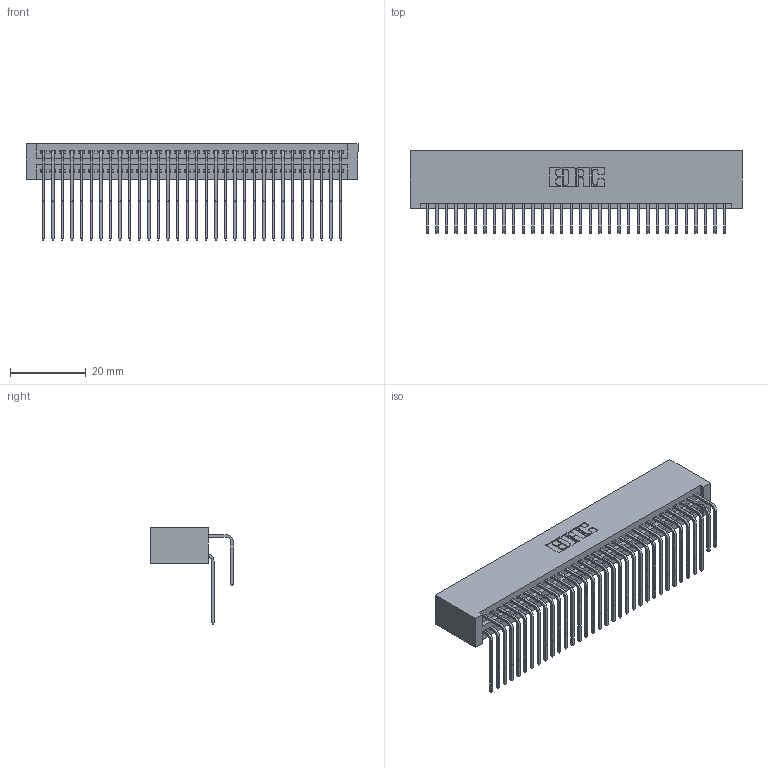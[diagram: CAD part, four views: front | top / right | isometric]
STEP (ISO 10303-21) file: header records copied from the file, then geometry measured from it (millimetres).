
FILE_DESCRIPTION (( 'STEP AP203' ), '1' );
FILE_NAME ('345-064-558-201.STEP', '2019-10-30T15:08:09', ( '' ), ( '' ), 'SwSTEP 2.0', 'SolidWorks 2016', '' );
FILE_SCHEMA (( 'CONFIG_CONTROL_DESIGN' ));
Length unit declared in the file: inch
Products named in the file (4): 345-292-001_558 Tail - 2; 345-292-001_558 559 Tail - 1; 345 Part_No Mounting Lugs; 345-064-558-201
Assembly tree (65 placements, depth 2):
  345-064-558-201
    345 Part_No Mounting Lugs
    345-292-001_558 559 Tail - 1  x32
    345-292-001_558 Tail - 2  x32
Bounding box: 87.88 x 21.83 x 25.53 mm (x, y, z)
Volume: 9429.4 mm3; surface area: 15784 mm2
Topology: 65 solids, 65 shells, 3446 faces, 10237 edges, 6738 vertices
Faces by surface type: plane 2316, cylinder 1130
Entity records: 27829 total; most frequent: CARTESIAN_POINT 4719, ORIENTED_EDGE 4602, DIRECTION 4141, EDGE_CURVE 2301, LINE 2009, VECTOR 2009, VERTEX_POINT 1530, AXIS2_PLACEMENT_3D 1066
